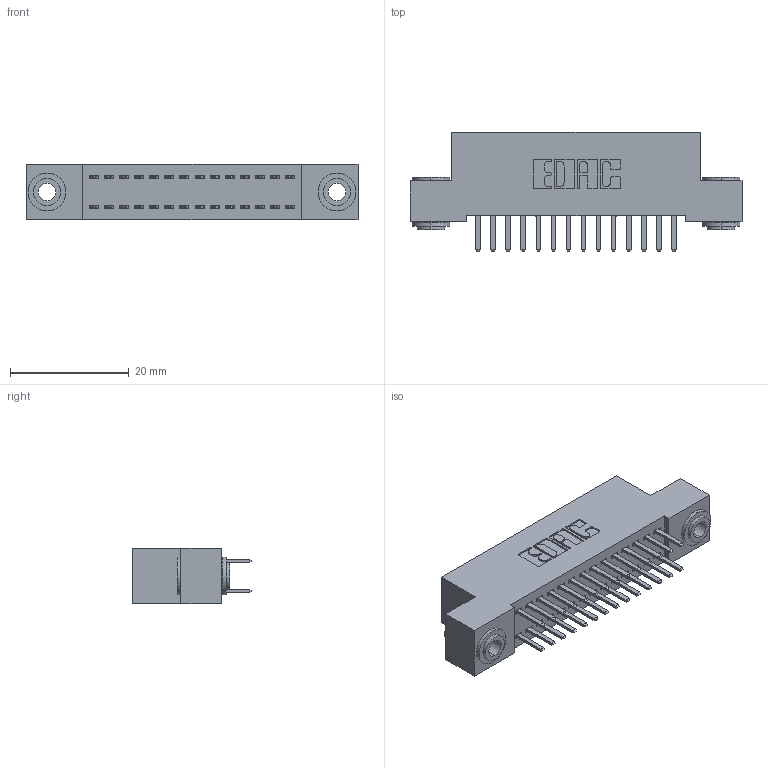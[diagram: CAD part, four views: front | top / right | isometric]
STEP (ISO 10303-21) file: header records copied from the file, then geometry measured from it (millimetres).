
FILE_DESCRIPTION (( 'STEP AP203' ), '1' );
FILE_NAME ('342-028-520-203.STEP', '2019-10-02T02:33:03', ( '' ), ( '' ), 'SwSTEP 2.0', 'SolidWorks 2016', '' );
FILE_SCHEMA (( 'CONFIG_CONTROL_DESIGN' ));
Length unit declared in the file: inch
Products named in the file (4): 342 Part_.156 TH; 345-292-001_345-293-120; 342-250-002_345-250-002-102; 342-028-520-203
Assembly tree (31 placements, depth 2):
  342-028-520-203
    342 Part_.156 TH
    345-292-001_345-293-120  x28
    342-250-002_345-250-002-102  x2
Bounding box: 55.88 x 20.02 x 9.4 mm (x, y, z)
Volume: 4898.8 mm3; surface area: 7469.1 mm2
Topology: 31 solids, 31 shells, 1716 faces, 4939 edges, 3214 vertices
Faces by surface type: plane 1140, cylinder 568, cone 8
Entity records: 13260 total; most frequent: CARTESIAN_POINT 2217, ORIENTED_EDGE 2134, DIRECTION 1965, EDGE_CURVE 1067, LINE 911, VECTOR 911, VERTEX_POINT 706, AXIS2_PLACEMENT_3D 527
